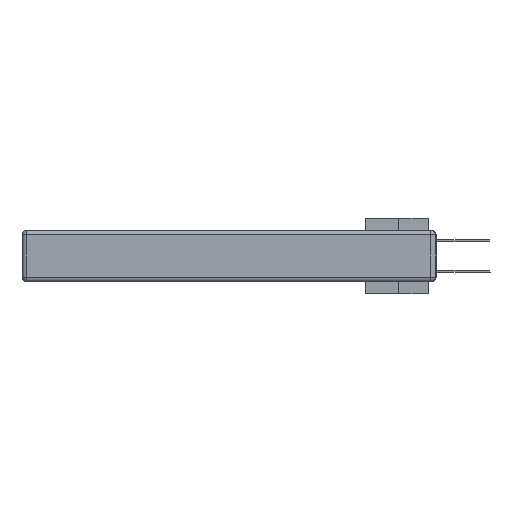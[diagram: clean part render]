
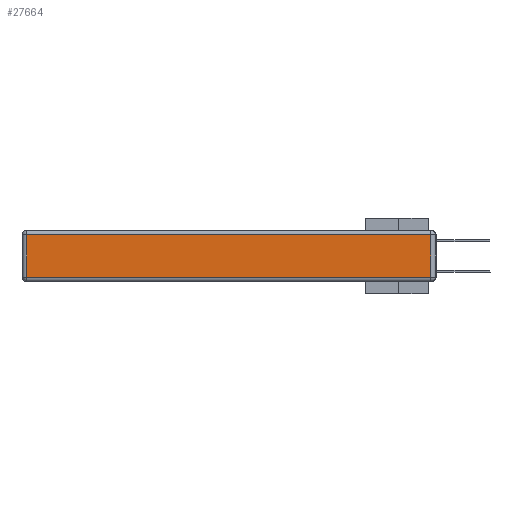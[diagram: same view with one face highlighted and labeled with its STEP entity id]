
A CAD part, left-side view. The second image highlights one B-rep face of the part: STEP entity #27664.
In plain terms, the highlighted planar face has unit normal (-1, 0, 0).
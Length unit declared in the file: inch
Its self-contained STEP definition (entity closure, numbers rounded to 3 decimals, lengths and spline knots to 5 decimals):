
#202 = CARTESIAN_POINT ( 'NONE',  ( 0., 0., -0.313 ) ) ;
#2207 = CARTESIAN_POINT ( 'NONE',  ( 0., 2.72, -0.313 ) ) ;
#3178 = LINE ( 'NONE', #202, #16931 ) ;
#3537 = DIRECTION ( 'NONE',  ( 0., 0., -1. ) ) ;
#4268 = CARTESIAN_POINT ( 'NONE',  ( 0., 0., -0.343 ) ) ;
#5759 = AXIS2_PLACEMENT_3D ( 'NONE', #4268, #22994, #23109 ) ;
#5784 = CARTESIAN_POINT ( 'NONE',  ( 0., 0.03, -0.343 ) ) ;
#7317 = PLANE ( 'NONE',  #5759 ) ;
#7417 = CARTESIAN_POINT ( 'NONE',  ( 0., 0.03, -0.03 ) ) ;
#8753 = ORIENTED_EDGE ( 'NONE', *, *, #34495, .T. ) ;
#11200 = VECTOR ( 'NONE', #3537, 39.37008 ) ;
#12891 = LINE ( 'NONE', #22046, #11200 ) ;
#14222 = LINE ( 'NONE', #26920, #25968 ) ;
#16423 = EDGE_CURVE ( 'NONE', #31841, #31421, #3178, .T. ) ;
#16424 = DIRECTION ( 'NONE',  ( 0., 0., 1. ) ) ;
#16931 = VECTOR ( 'NONE', #27010, 39.37008 ) ;
#17379 = ORIENTED_EDGE ( 'NONE', *, *, #16423, .T. ) ;
#18445 = CARTESIAN_POINT ( 'NONE',  ( 0., 2.72, -0.03 ) ) ;
#20899 = VERTEX_POINT ( 'NONE', #7417 ) ;
#22046 = CARTESIAN_POINT ( 'NONE',  ( 0., 2.72, -0.343 ) ) ;
#22730 = LINE ( 'NONE', #5784, #24412 ) ;
#22763 = ORIENTED_EDGE ( 'NONE', *, *, #30889, .T. ) ;
#22994 = DIRECTION ( 'NONE',  ( -1., 0., 0. ) ) ;
#23109 = DIRECTION ( 'NONE',  ( 0., 0., 1. ) ) ;
#23419 = VERTEX_POINT ( 'NONE', #18445 ) ;
#23509 = EDGE_LOOP ( 'NONE', ( #17379, #22763, #33626, #8753 ) ) ;
#24412 = VECTOR ( 'NONE', #16424, 39.37008 ) ;
#24581 = DIRECTION ( 'NONE',  ( 0., 1., 0. ) ) ;
#25968 = VECTOR ( 'NONE', #24581, 39.37008 ) ;
#26920 = CARTESIAN_POINT ( 'NONE',  ( 0., 2.75, -0.03 ) ) ;
#27010 = DIRECTION ( 'NONE',  ( 0., -1., 0. ) ) ;
#27664 = ADVANCED_FACE ( 'NONE', ( #29456 ), #7317, .T. ) ;
#29456 = FACE_OUTER_BOUND ( 'NONE', #23509, .T. ) ;
#30889 = EDGE_CURVE ( 'NONE', #31421, #20899, #22730, .T. ) ;
#31421 = VERTEX_POINT ( 'NONE', #31860 ) ;
#31841 = VERTEX_POINT ( 'NONE', #2207 ) ;
#31860 = CARTESIAN_POINT ( 'NONE',  ( 0., 0.03, -0.313 ) ) ;
#33197 = EDGE_CURVE ( 'NONE', #20899, #23419, #14222, .T. ) ;
#33626 = ORIENTED_EDGE ( 'NONE', *, *, #33197, .T. ) ;
#34495 = EDGE_CURVE ( 'NONE', #23419, #31841, #12891, .T. ) ;
